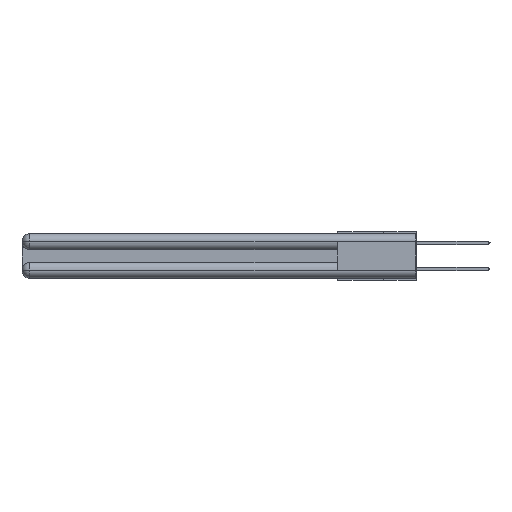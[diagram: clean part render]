
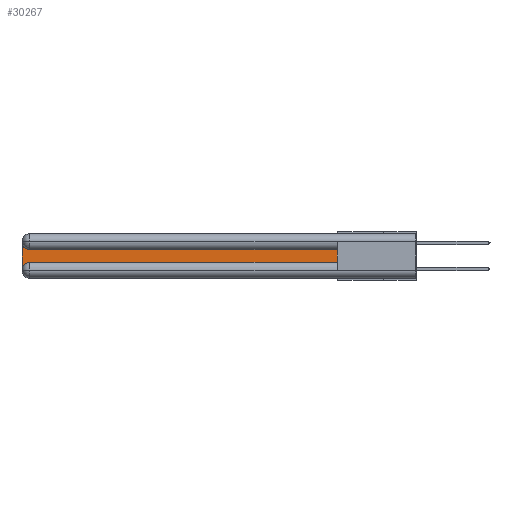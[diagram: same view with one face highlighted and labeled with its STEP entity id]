
A CAD part, left-side view. The second image highlights one B-rep face of the part: STEP entity #30267.
In plain terms, the highlighted planar face has unit normal (-1, 0, 0).
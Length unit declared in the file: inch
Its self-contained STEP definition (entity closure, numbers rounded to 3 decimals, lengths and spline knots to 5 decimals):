
#90 = LINE ( 'NONE', #20030, #15877 ) ;
#212 = CARTESIAN_POINT ( 'NONE',  ( 0.075, 0.6, -0.1225 ) ) ;
#327 = CARTESIAN_POINT ( 'NONE',  ( 0.075, 3., -0.1225 ) ) ;
#418 = EDGE_CURVE ( 'NONE', #20455, #17093, #90, .T. ) ;
#1449 = FACE_OUTER_BOUND ( 'NONE', #16350, .T. ) ;
#3052 = LINE ( 'NONE', #21138, #8971 ) ;
#3291 = EDGE_CURVE ( 'NONE', #25176, #32009, #3052, .T. ) ;
#3433 = ORIENTED_EDGE ( 'NONE', *, *, #3291, .T. ) ;
#4398 = DIRECTION ( 'NONE',  ( 0., 0., 1. ) ) ;
#4427 = CARTESIAN_POINT ( 'NONE',  ( 0.075, 2.94, -0.2775 ) ) ;
#4743 = DIRECTION ( 'NONE',  ( 1., 0., 0. ) ) ;
#5636 = DIRECTION ( 'NONE',  ( 0., 0., -1. ) ) ;
#6017 = VECTOR ( 'NONE', #4398, 39.37008 ) ;
#6085 = ORIENTED_EDGE ( 'NONE', *, *, #6260, .T. ) ;
#6260 = EDGE_CURVE ( 'NONE', #32009, #18304, #12721, .T. ) ;
#7511 = CARTESIAN_POINT ( 'NONE',  ( 0.075, 2.94, -0.1225 ) ) ;
#8153 = VERTEX_POINT ( 'NONE', #7511 ) ;
#8769 = EDGE_CURVE ( 'NONE', #8153, #20455, #32652, .T. ) ;
#8895 = VECTOR ( 'NONE', #15911, 39.37008 ) ;
#8971 = VECTOR ( 'NONE', #28618, 39.37008 ) ;
#9598 = DIRECTION ( 'NONE',  ( 0., 0., -1. ) ) ;
#9989 = CARTESIAN_POINT ( 'NONE',  ( 0.075, 2.94, -0.2175 ) ) ;
#12721 = LINE ( 'NONE', #24627, #6017 ) ;
#12913 = CARTESIAN_POINT ( 'NONE',  ( 0.075, 3., -0.2775 ) ) ;
#15344 = DIRECTION ( 'NONE',  ( 0., 0., -1. ) ) ;
#15877 = VECTOR ( 'NONE', #19804, 39.37008 ) ;
#15911 = DIRECTION ( 'NONE',  ( 0., 1., 0. ) ) ;
#16350 = EDGE_LOOP ( 'NONE', ( #25642, #29507, #19052, #31261, #3433, #6085 ) ) ;
#16868 = CIRCLE ( 'NONE', #22728, 0.06 ) ;
#17093 = VERTEX_POINT ( 'NONE', #12913 ) ;
#18304 = VERTEX_POINT ( 'NONE', #212 ) ;
#19052 = ORIENTED_EDGE ( 'NONE', *, *, #418, .T. ) ;
#19804 = DIRECTION ( 'NONE',  ( 0., 0., -1. ) ) ;
#20030 = CARTESIAN_POINT ( 'NONE',  ( 0.075, 3., -0.2175 ) ) ;
#20244 = CARTESIAN_POINT ( 'NONE',  ( 0.075, 2.94, -0.0625 ) ) ;
#20359 = EDGE_CURVE ( 'NONE', #17093, #25176, #16868, .T. ) ;
#20455 = VERTEX_POINT ( 'NONE', #27661 ) ;
#20539 = PLANE ( 'NONE',  #27199 ) ;
#21138 = CARTESIAN_POINT ( 'NONE',  ( 0.075, 0.6, -0.2175 ) ) ;
#22728 = AXIS2_PLACEMENT_3D ( 'NONE', #4427, #4743, #9598 ) ;
#22904 = DIRECTION ( 'NONE',  ( 1., 0., 0. ) ) ;
#23087 = DIRECTION ( 'NONE',  ( 1., 0., 0. ) ) ;
#24627 = CARTESIAN_POINT ( 'NONE',  ( 0.075, 0.6, -0.2175 ) ) ;
#25176 = VERTEX_POINT ( 'NONE', #9989 ) ;
#25642 = ORIENTED_EDGE ( 'NONE', *, *, #31476, .T. ) ;
#26264 = LINE ( 'NONE', #28271, #8895 ) ;
#27199 = AXIS2_PLACEMENT_3D ( 'NONE', #327, #23087, #5636 ) ;
#27661 = CARTESIAN_POINT ( 'NONE',  ( 0.075, 3., -0.0625 ) ) ;
#28271 = CARTESIAN_POINT ( 'NONE',  ( 0.075, 0.6, -0.1225 ) ) ;
#28618 = DIRECTION ( 'NONE',  ( 0., -1., 0. ) ) ;
#29507 = ORIENTED_EDGE ( 'NONE', *, *, #8769, .T. ) ;
#30267 = ADVANCED_FACE ( 'NONE', ( #1449 ), #20539, .F. ) ;
#31237 = CARTESIAN_POINT ( 'NONE',  ( 0.075, 0.6, -0.2175 ) ) ;
#31261 = ORIENTED_EDGE ( 'NONE', *, *, #20359, .T. ) ;
#31425 = AXIS2_PLACEMENT_3D ( 'NONE', #20244, #22904, #15344 ) ;
#31476 = EDGE_CURVE ( 'NONE', #18304, #8153, #26264, .T. ) ;
#32009 = VERTEX_POINT ( 'NONE', #31237 ) ;
#32652 = CIRCLE ( 'NONE', #31425, 0.06 ) ;
